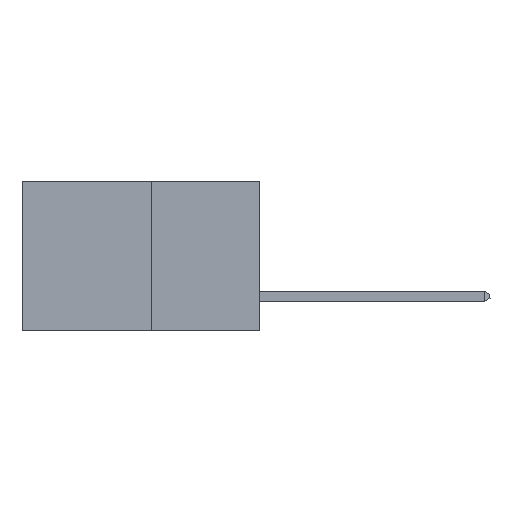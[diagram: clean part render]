
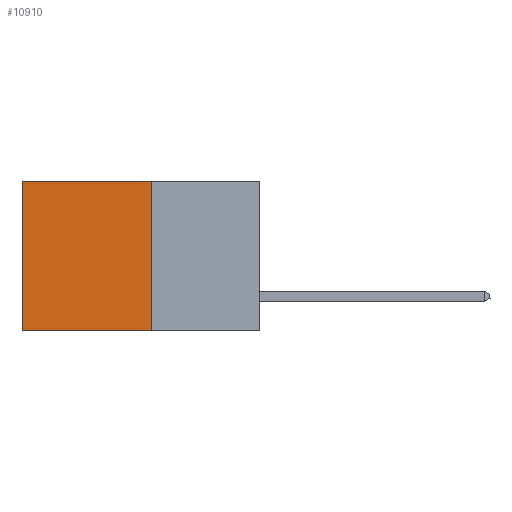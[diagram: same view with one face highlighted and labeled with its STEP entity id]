
A CAD part, left-side view. The second image highlights one B-rep face of the part: STEP entity #10910.
In plain terms, the highlighted planar face has unit normal (-1, 0, 0).
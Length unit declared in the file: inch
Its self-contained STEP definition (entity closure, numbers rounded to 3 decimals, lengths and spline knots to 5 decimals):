
#331 = VERTEX_POINT ( 'NONE', #5692 ) ;
#603 = CARTESIAN_POINT ( 'NONE',  ( 0.277, 0.27, 0. ) ) ;
#670 = FACE_OUTER_BOUND ( 'NONE', #6649, .T. ) ;
#790 = EDGE_CURVE ( 'NONE', #1048, #331, #2572, .T. ) ;
#1048 = VERTEX_POINT ( 'NONE', #603 ) ;
#1066 = VECTOR ( 'NONE', #1244, 39.37008 ) ;
#1244 = DIRECTION ( 'NONE',  ( 0., 1., 0. ) ) ;
#2099 = VERTEX_POINT ( 'NONE', #9364 ) ;
#2572 = LINE ( 'NONE', #3762, #13185 ) ;
#3271 = DIRECTION ( 'NONE',  ( 0., 0., -1. ) ) ;
#3554 = EDGE_CURVE ( 'NONE', #2099, #12863, #6787, .T. ) ;
#3667 = VECTOR ( 'NONE', #9005, 39.37008 ) ;
#3762 = CARTESIAN_POINT ( 'NONE',  ( 0.277, 0.27, -0.37 ) ) ;
#3798 = CARTESIAN_POINT ( 'NONE',  ( 0.277, 0.27, -0.37 ) ) ;
#4570 = AXIS2_PLACEMENT_3D ( 'NONE', #3798, #11037, #4845 ) ;
#4602 = EDGE_CURVE ( 'NONE', #331, #12863, #9463, .T. ) ;
#4845 = DIRECTION ( 'NONE',  ( 0., 0., -1. ) ) ;
#4993 = ORIENTED_EDGE ( 'NONE', *, *, #4602, .F. ) ;
#4997 = ORIENTED_EDGE ( 'NONE', *, *, #790, .F. ) ;
#5118 = ORIENTED_EDGE ( 'NONE', *, *, #3554, .T. ) ;
#5692 = CARTESIAN_POINT ( 'NONE',  ( 0.277, 0.27, -0.37 ) ) ;
#6126 = CARTESIAN_POINT ( 'NONE',  ( 0.277, 0.59, -0.37 ) ) ;
#6649 = EDGE_LOOP ( 'NONE', ( #5118, #4993, #4997, #12596 ) ) ;
#6787 = LINE ( 'NONE', #6126, #3667 ) ;
#7354 = LINE ( 'NONE', #8914, #12759 ) ;
#7922 = CARTESIAN_POINT ( 'NONE',  ( 0.277, 0.27, -0.37 ) ) ;
#8914 = CARTESIAN_POINT ( 'NONE',  ( 0.277, 0.27, 0. ) ) ;
#9005 = DIRECTION ( 'NONE',  ( 0., 0., -1. ) ) ;
#9364 = CARTESIAN_POINT ( 'NONE',  ( 0.277, 0.59, 0. ) ) ;
#9463 = LINE ( 'NONE', #7922, #1066 ) ;
#9977 = DIRECTION ( 'NONE',  ( 0., 1., 0. ) ) ;
#10046 = CARTESIAN_POINT ( 'NONE',  ( 0.277, 0.59, -0.37 ) ) ;
#10388 = EDGE_CURVE ( 'NONE', #1048, #2099, #7354, .T. ) ;
#10910 = ADVANCED_FACE ( 'NONE', ( #670 ), #10987, .F. ) ;
#10987 = PLANE ( 'NONE',  #4570 ) ;
#11037 = DIRECTION ( 'NONE',  ( 1., 0., 0. ) ) ;
#12596 = ORIENTED_EDGE ( 'NONE', *, *, #10388, .T. ) ;
#12759 = VECTOR ( 'NONE', #9977, 39.37008 ) ;
#12863 = VERTEX_POINT ( 'NONE', #10046 ) ;
#13185 = VECTOR ( 'NONE', #3271, 39.37008 ) ;
